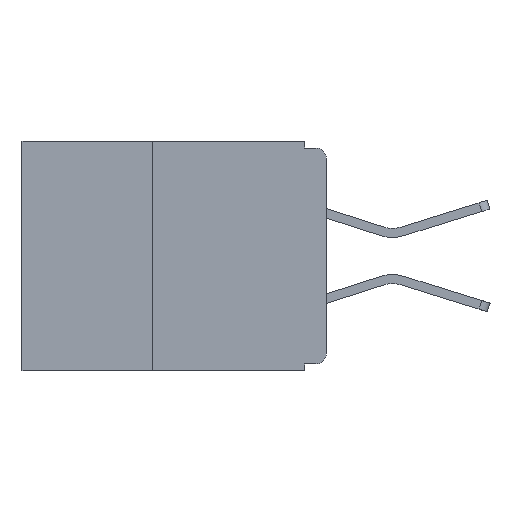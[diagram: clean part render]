
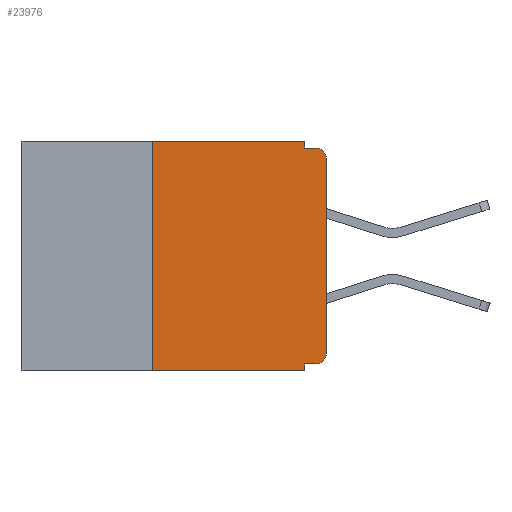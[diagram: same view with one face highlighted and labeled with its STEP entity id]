
A CAD part, left-side view. The second image highlights one B-rep face of the part: STEP entity #23976.
In plain terms, the highlighted planar face has unit normal (-1, 0, 0).
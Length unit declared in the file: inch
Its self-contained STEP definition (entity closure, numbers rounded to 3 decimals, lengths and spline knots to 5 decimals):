
#1256 = DIRECTION ( 'NONE',  ( 1., 0., 0. ) ) ;
#1943 = CARTESIAN_POINT ( 'NONE',  ( 0., 0.015, -0.025 ) ) ;
#2827 = VERTEX_POINT ( 'NONE', #30679 ) ;
#3110 = ORIENTED_EDGE ( 'NONE', *, *, #12129, .T. ) ;
#3130 = LINE ( 'NONE', #33574, #9434 ) ;
#3501 = ORIENTED_EDGE ( 'NONE', *, *, #17339, .T. ) ;
#4156 = CARTESIAN_POINT ( 'NONE',  ( 0., 0.031, 0. ) ) ;
#4275 = DIRECTION ( 'NONE',  ( 0., 0., -1. ) ) ;
#4645 = DIRECTION ( 'NONE',  ( 0., 0., -1. ) ) ;
#4649 = CARTESIAN_POINT ( 'NONE',  ( 0., 0.015, -0.305 ) ) ;
#4894 = LINE ( 'NONE', #4156, #32828 ) ;
#4952 = VECTOR ( 'NONE', #8875, 39.37008 ) ;
#5265 = VERTEX_POINT ( 'NONE', #26356 ) ;
#5613 = AXIS2_PLACEMENT_3D ( 'NONE', #4649, #23181, #7367 ) ;
#5777 = LINE ( 'NONE', #9108, #9532 ) ;
#5797 = LINE ( 'NONE', #22136, #4952 ) ;
#6067 = ORIENTED_EDGE ( 'NONE', *, *, #7235, .F. ) ;
#6288 = DIRECTION ( 'NONE',  ( 0., -1., 0. ) ) ;
#6824 = VERTEX_POINT ( 'NONE', #13065 ) ;
#7235 = EDGE_CURVE ( 'NONE', #6824, #11281, #4894, .T. ) ;
#7367 = DIRECTION ( 'NONE',  ( 0., 0., -1. ) ) ;
#7508 = ORIENTED_EDGE ( 'NONE', *, *, #9061, .F. ) ;
#7914 = CARTESIAN_POINT ( 'NONE',  ( 0., 0.437, 0. ) ) ;
#8517 = DIRECTION ( 'NONE',  ( 0., 0., 1. ) ) ;
#8655 = CARTESIAN_POINT ( 'NONE',  ( 0., 0.25, -0.33 ) ) ;
#8759 = LINE ( 'NONE', #28686, #28086 ) ;
#8849 = CIRCLE ( 'NONE', #19501, 0.015 ) ;
#8875 = DIRECTION ( 'NONE',  ( 0., 1., 0. ) ) ;
#9061 = EDGE_CURVE ( 'NONE', #20953, #15986, #22209, .T. ) ;
#9108 = CARTESIAN_POINT ( 'NONE',  ( 0., 0.031, -0.33 ) ) ;
#9434 = VECTOR ( 'NONE', #23295, 39.37008 ) ;
#9532 = VECTOR ( 'NONE', #30129, 39.37008 ) ;
#9755 = EDGE_CURVE ( 'NONE', #15986, #6824, #21734, .T. ) ;
#11201 = CARTESIAN_POINT ( 'NONE',  ( 0., 0.031, -0.01 ) ) ;
#11281 = VERTEX_POINT ( 'NONE', #11201 ) ;
#11405 = CARTESIAN_POINT ( 'NONE',  ( 0., 0.25, -0.33 ) ) ;
#12129 = EDGE_CURVE ( 'NONE', #5265, #19156, #28934, .T. ) ;
#12918 = DIRECTION ( 'NONE',  ( 0., 0., 1. ) ) ;
#13065 = CARTESIAN_POINT ( 'NONE',  ( 0., 0.031, 0. ) ) ;
#13186 = CARTESIAN_POINT ( 'NONE',  ( 0., 0.031, -0.32 ) ) ;
#14847 = CARTESIAN_POINT ( 'NONE',  ( 0., 0., -0.305 ) ) ;
#14876 = EDGE_LOOP ( 'NONE', ( #16809, #3501, #24632, #6067, #32345, #7508, #23603, #22612, #15582, #3110 ) ) ;
#15148 = CARTESIAN_POINT ( 'NONE',  ( 0., 0., -0.01 ) ) ;
#15170 = VECTOR ( 'NONE', #8517, 39.37008 ) ;
#15352 = FACE_OUTER_BOUND ( 'NONE', #14876, .T. ) ;
#15582 = ORIENTED_EDGE ( 'NONE', *, *, #19049, .F. ) ;
#15986 = VERTEX_POINT ( 'NONE', #21903 ) ;
#16809 = ORIENTED_EDGE ( 'NONE', *, *, #18733, .T. ) ;
#17339 = EDGE_CURVE ( 'NONE', #20594, #24558, #8849, .T. ) ;
#18733 = EDGE_CURVE ( 'NONE', #19156, #20594, #8759, .T. ) ;
#19049 = EDGE_CURVE ( 'NONE', #5265, #27531, #5797, .T. ) ;
#19156 = VERTEX_POINT ( 'NONE', #14847 ) ;
#19501 = AXIS2_PLACEMENT_3D ( 'NONE', #1943, #20512, #4645 ) ;
#19845 = DIRECTION ( 'NONE',  ( 0., 0., -1. ) ) ;
#20512 = DIRECTION ( 'NONE',  ( -1., 0., 0. ) ) ;
#20594 = VERTEX_POINT ( 'NONE', #30301 ) ;
#20953 = VERTEX_POINT ( 'NONE', #11405 ) ;
#21734 = LINE ( 'NONE', #7914, #33890 ) ;
#21903 = CARTESIAN_POINT ( 'NONE',  ( 0., 0.25, 0. ) ) ;
#22136 = CARTESIAN_POINT ( 'NONE',  ( 0., 0., -0.32 ) ) ;
#22209 = LINE ( 'NONE', #8655, #15170 ) ;
#22400 = PLANE ( 'NONE',  #29131 ) ;
#22423 = VECTOR ( 'NONE', #28382, 39.37008 ) ;
#22612 = ORIENTED_EDGE ( 'NONE', *, *, #33883, .F. ) ;
#23181 = DIRECTION ( 'NONE',  ( -1., 0., 0. ) ) ;
#23262 = LINE ( 'NONE', #15148, #22423 ) ;
#23295 = DIRECTION ( 'NONE',  ( 0., -1., 0. ) ) ;
#23513 = EDGE_CURVE ( 'NONE', #11281, #24558, #23262, .T. ) ;
#23603 = ORIENTED_EDGE ( 'NONE', *, *, #26292, .T. ) ;
#23976 = ADVANCED_FACE ( 'NONE', ( #15352 ), #22400, .F. ) ;
#24558 = VERTEX_POINT ( 'NONE', #27978 ) ;
#24632 = ORIENTED_EDGE ( 'NONE', *, *, #23513, .F. ) ;
#26292 = EDGE_CURVE ( 'NONE', #20953, #2827, #3130, .T. ) ;
#26356 = CARTESIAN_POINT ( 'NONE',  ( 0., 0.015, -0.32 ) ) ;
#27531 = VERTEX_POINT ( 'NONE', #13186 ) ;
#27978 = CARTESIAN_POINT ( 'NONE',  ( 0., 0.015, -0.01 ) ) ;
#28086 = VECTOR ( 'NONE', #12918, 39.37008 ) ;
#28382 = DIRECTION ( 'NONE',  ( 0., -1., 0. ) ) ;
#28686 = CARTESIAN_POINT ( 'NONE',  ( 0., 0., 0. ) ) ;
#28934 = CIRCLE ( 'NONE', #5613, 0.015 ) ;
#29131 = AXIS2_PLACEMENT_3D ( 'NONE', #30281, #1256, #19845 ) ;
#30129 = DIRECTION ( 'NONE',  ( 0., 0., -1. ) ) ;
#30281 = CARTESIAN_POINT ( 'NONE',  ( 0., 0.437, 0. ) ) ;
#30301 = CARTESIAN_POINT ( 'NONE',  ( 0., 0., -0.025 ) ) ;
#30679 = CARTESIAN_POINT ( 'NONE',  ( 0., 0.031, -0.33 ) ) ;
#32345 = ORIENTED_EDGE ( 'NONE', *, *, #9755, .F. ) ;
#32828 = VECTOR ( 'NONE', #4275, 39.37008 ) ;
#33574 = CARTESIAN_POINT ( 'NONE',  ( 0., 0.437, -0.33 ) ) ;
#33883 = EDGE_CURVE ( 'NONE', #27531, #2827, #5777, .T. ) ;
#33890 = VECTOR ( 'NONE', #6288, 39.37008 ) ;
